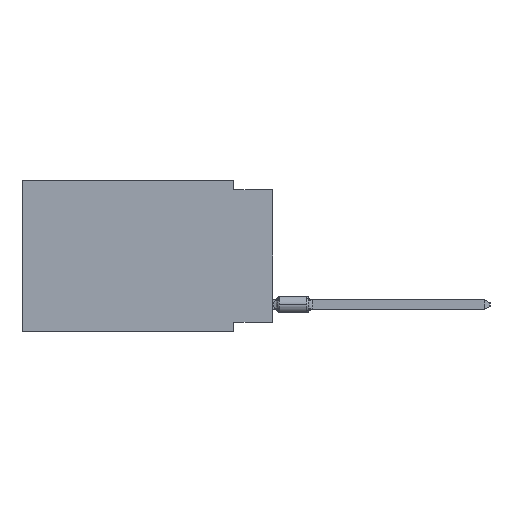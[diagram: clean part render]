
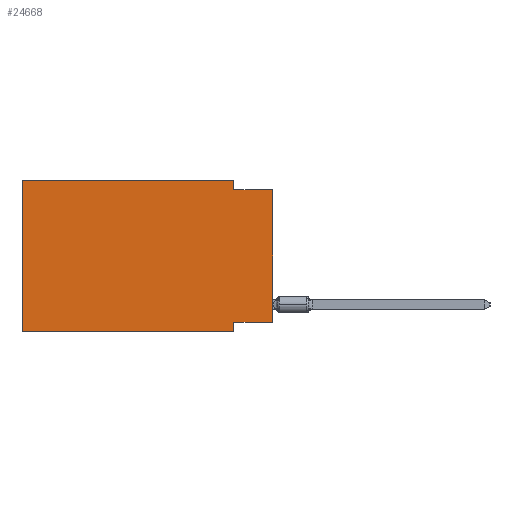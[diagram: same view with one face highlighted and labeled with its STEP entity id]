
A CAD part, left-side view. The second image highlights one B-rep face of the part: STEP entity #24668.
In plain terms, the highlighted planar face has unit normal (-1, 0, 0).
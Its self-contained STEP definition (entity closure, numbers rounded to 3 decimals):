
#604 = LINE ( 'NONE', #20162, #10104 ) ;
#828 = VECTOR ( 'NONE', #15545, 1000. ) ;
#1381 = DIRECTION ( 'NONE',  ( 0., -1., 0. ) ) ;
#1781 = CARTESIAN_POINT ( 'NONE',  ( 0., 2.54, -0.635 ) ) ;
#3617 = ORIENTED_EDGE ( 'NONE', *, *, #7207, .T. ) ;
#4751 = VERTEX_POINT ( 'NONE', #20936 ) ;
#4889 = EDGE_CURVE ( 'NONE', #15936, #22531, #34803, .T. ) ;
#5303 = ORIENTED_EDGE ( 'NONE', *, *, #35659, .F. ) ;
#5396 = LINE ( 'NONE', #20734, #25570 ) ;
#6226 = CARTESIAN_POINT ( 'NONE',  ( 0., 16.383, 0. ) ) ;
#6790 = VECTOR ( 'NONE', #1381, 1000. ) ;
#6902 = ORIENTED_EDGE ( 'NONE', *, *, #29727, .F. ) ;
#7207 = EDGE_CURVE ( 'NONE', #35382, #42344, #7498, .T. ) ;
#7498 = LINE ( 'NONE', #27236, #21015 ) ;
#8323 = EDGE_CURVE ( 'NONE', #32567, #36294, #22500, .T. ) ;
#9919 = AXIS2_PLACEMENT_3D ( 'NONE', #10319, #27235, #10107 ) ;
#10104 = VECTOR ( 'NONE', #37284, 1000. ) ;
#10107 = DIRECTION ( 'NONE',  ( 0., 0., -1. ) ) ;
#10319 = CARTESIAN_POINT ( 'NONE',  ( 0., 16.383, 0. ) ) ;
#10511 = EDGE_LOOP ( 'NONE', ( #26014, #31562, #28965, #13955, #5303, #3617, #12641, #6902 ) ) ;
#10953 = PLANE ( 'NONE',  #9919 ) ;
#11143 = LINE ( 'NONE', #28071, #39328 ) ;
#11598 = CARTESIAN_POINT ( 'NONE',  ( 0., 2.54, -9.906 ) ) ;
#12026 = DIRECTION ( 'NONE',  ( 0., 0., -1. ) ) ;
#12504 = CARTESIAN_POINT ( 'NONE',  ( 0., 16.383, 0. ) ) ;
#12641 = ORIENTED_EDGE ( 'NONE', *, *, #30291, .F. ) ;
#13955 = ORIENTED_EDGE ( 'NONE', *, *, #8323, .F. ) ;
#15545 = DIRECTION ( 'NONE',  ( 0., -1., 0. ) ) ;
#15936 = VERTEX_POINT ( 'NONE', #1781 ) ;
#16847 = DIRECTION ( 'NONE',  ( 0., 0., -1. ) ) ;
#17348 = CARTESIAN_POINT ( 'NONE',  ( 0., 16.383, 0. ) ) ;
#18517 = EDGE_CURVE ( 'NONE', #36294, #15936, #5396, .T. ) ;
#19463 = DIRECTION ( 'NONE',  ( 0., 0., 1. ) ) ;
#20091 = FACE_OUTER_BOUND ( 'NONE', #10511, .T. ) ;
#20162 = CARTESIAN_POINT ( 'NONE',  ( 0., 0., -9.271 ) ) ;
#20734 = CARTESIAN_POINT ( 'NONE',  ( 0., 2.54, 0. ) ) ;
#20936 = CARTESIAN_POINT ( 'NONE',  ( 0., 2.54, -9.271 ) ) ;
#21015 = VECTOR ( 'NONE', #40263, 1000. ) ;
#21372 = LINE ( 'NONE', #11598, #37153 ) ;
#21555 = DIRECTION ( 'NONE',  ( 0., 0., 1. ) ) ;
#22170 = EDGE_CURVE ( 'NONE', #40840, #22531, #11143, .T. ) ;
#22500 = LINE ( 'NONE', #12504, #828 ) ;
#22531 = VERTEX_POINT ( 'NONE', #37369 ) ;
#22584 = CARTESIAN_POINT ( 'NONE',  ( 0., 2.54, -9.906 ) ) ;
#22908 = VECTOR ( 'NONE', #19463, 1000. ) ;
#23019 = CARTESIAN_POINT ( 'NONE',  ( 0., 16.383, -9.906 ) ) ;
#23476 = CARTESIAN_POINT ( 'NONE',  ( 0., 0., -9.271 ) ) ;
#24668 = ADVANCED_FACE ( 'NONE', ( #20091 ), #10953, .F. ) ;
#25570 = VECTOR ( 'NONE', #16847, 1000. ) ;
#26014 = ORIENTED_EDGE ( 'NONE', *, *, #22170, .T. ) ;
#27235 = DIRECTION ( 'NONE',  ( 1., 0., 0. ) ) ;
#27236 = CARTESIAN_POINT ( 'NONE',  ( 0., 16.383, -9.906 ) ) ;
#28071 = CARTESIAN_POINT ( 'NONE',  ( 0., 0., 0. ) ) ;
#28965 = ORIENTED_EDGE ( 'NONE', *, *, #18517, .F. ) ;
#29727 = EDGE_CURVE ( 'NONE', #40840, #4751, #604, .T. ) ;
#30175 = CARTESIAN_POINT ( 'NONE',  ( 0., 2.54, 0. ) ) ;
#30291 = EDGE_CURVE ( 'NONE', #4751, #42344, #21372, .T. ) ;
#31562 = ORIENTED_EDGE ( 'NONE', *, *, #4889, .F. ) ;
#32567 = VERTEX_POINT ( 'NONE', #17348 ) ;
#34803 = LINE ( 'NONE', #41106, #6790 ) ;
#35382 = VERTEX_POINT ( 'NONE', #23019 ) ;
#35659 = EDGE_CURVE ( 'NONE', #35382, #32567, #35964, .T. ) ;
#35964 = LINE ( 'NONE', #6226, #22908 ) ;
#36294 = VERTEX_POINT ( 'NONE', #30175 ) ;
#37153 = VECTOR ( 'NONE', #12026, 1000. ) ;
#37284 = DIRECTION ( 'NONE',  ( 0., 1., 0. ) ) ;
#37369 = CARTESIAN_POINT ( 'NONE',  ( 0., 0., -0.635 ) ) ;
#39328 = VECTOR ( 'NONE', #21555, 1000. ) ;
#40263 = DIRECTION ( 'NONE',  ( 0., -1., 0. ) ) ;
#40840 = VERTEX_POINT ( 'NONE', #23476 ) ;
#41106 = CARTESIAN_POINT ( 'NONE',  ( 0., 0., -0.635 ) ) ;
#42344 = VERTEX_POINT ( 'NONE', #22584 ) ;
